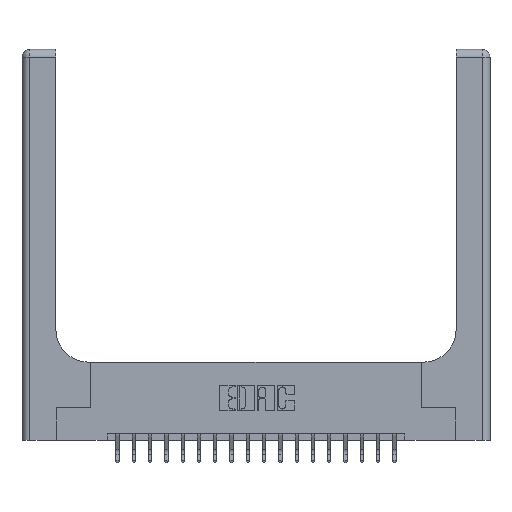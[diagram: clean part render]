
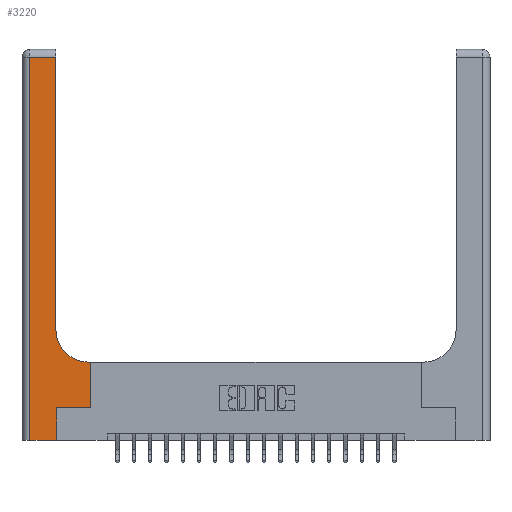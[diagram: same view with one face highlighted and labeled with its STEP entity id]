
A CAD part, top view. The second image highlights one B-rep face of the part: STEP entity #3220.
In plain terms, the highlighted planar face has unit normal (0, 0, 1).
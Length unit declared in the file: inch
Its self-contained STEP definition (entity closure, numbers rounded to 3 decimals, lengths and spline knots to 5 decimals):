
#283 = VERTEX_POINT ( 'NONE', #16008 ) ;
#293 = CARTESIAN_POINT ( 'NONE',  ( 0.51, 0.6, 0.37 ) ) ;
#525 = DIRECTION ( 'NONE',  ( 1., 0., 0. ) ) ;
#760 = DIRECTION ( 'NONE',  ( -1., 0., 0. ) ) ;
#823 = VECTOR ( 'NONE', #4569, 39.37008 ) ;
#890 = EDGE_CURVE ( 'NONE', #11549, #8494, #15449, .T. ) ;
#1393 = EDGE_CURVE ( 'NONE', #13385, #9423, #1812, .T. ) ;
#1415 = DIRECTION ( 'NONE',  ( 1., 0., 0. ) ) ;
#1431 = CARTESIAN_POINT ( 'NONE',  ( 0., 2.94, 0.37 ) ) ;
#1812 = LINE ( 'NONE', #1431, #823 ) ;
#2253 = CIRCLE ( 'NONE', #16131, 0.25 ) ;
#2894 = DIRECTION ( 'NONE',  ( 0., 1., 0. ) ) ;
#3220 = ADVANCED_FACE ( 'NONE', ( #13397 ), #10741, .F. ) ;
#3382 = LINE ( 'NONE', #13489, #16966 ) ;
#3398 = EDGE_CURVE ( 'NONE', #19363, #19264, #2253, .T. ) ;
#3534 = CARTESIAN_POINT ( 'NONE',  ( 0.26, 2.94, 0.37 ) ) ;
#3695 = VECTOR ( 'NONE', #13557, 39.37008 ) ;
#4569 = DIRECTION ( 'NONE',  ( -1., 0., 0. ) ) ;
#5801 = CARTESIAN_POINT ( 'NONE',  ( 0., 3., 0.37 ) ) ;
#6006 = DIRECTION ( 'NONE',  ( 0., 0., -1. ) ) ;
#6201 = CARTESIAN_POINT ( 'NONE',  ( 0., 0., 0.37 ) ) ;
#6215 = DIRECTION ( 'NONE',  ( 1., 0., 0. ) ) ;
#6959 = EDGE_CURVE ( 'NONE', #8494, #16603, #14528, .T. ) ;
#7045 = ORIENTED_EDGE ( 'NONE', *, *, #890, .T. ) ;
#7109 = CARTESIAN_POINT ( 'NONE',  ( 0.06, 3., 0.37 ) ) ;
#7228 = VECTOR ( 'NONE', #17967, 39.37008 ) ;
#7435 = CARTESIAN_POINT ( 'NONE',  ( 0.528, 0.25, 0.37 ) ) ;
#7507 = VECTOR ( 'NONE', #10739, 39.37008 ) ;
#7674 = EDGE_CURVE ( 'NONE', #8928, #11549, #9984, .T. ) ;
#8494 = VERTEX_POINT ( 'NONE', #15177 ) ;
#8783 = VECTOR ( 'NONE', #1415, 39.37008 ) ;
#8928 = VERTEX_POINT ( 'NONE', #9923 ) ;
#9072 = ORIENTED_EDGE ( 'NONE', *, *, #3398, .T. ) ;
#9423 = VERTEX_POINT ( 'NONE', #20302 ) ;
#9435 = CARTESIAN_POINT ( 'NONE',  ( 0.26, 3., 0.37 ) ) ;
#9743 = EDGE_CURVE ( 'NONE', #9423, #283, #19953, .T. ) ;
#9748 = ORIENTED_EDGE ( 'NONE', *, *, #1393, .T. ) ;
#9895 = CARTESIAN_POINT ( 'NONE',  ( 0.265, 0., 0.37 ) ) ;
#9923 = CARTESIAN_POINT ( 'NONE',  ( 0.265, 0., 0.37 ) ) ;
#9984 = LINE ( 'NONE', #9895, #7228 ) ;
#10601 = DIRECTION ( 'NONE',  ( -1., 0., 0. ) ) ;
#10739 = DIRECTION ( 'NONE',  ( 0., 1., 0. ) ) ;
#10741 = PLANE ( 'NONE',  #14442 ) ;
#11025 = EDGE_CURVE ( 'NONE', #19264, #13385, #14865, .T. ) ;
#11232 = VECTOR ( 'NONE', #525, 39.37008 ) ;
#11294 = ORIENTED_EDGE ( 'NONE', *, *, #9743, .T. ) ;
#11509 = CARTESIAN_POINT ( 'NONE',  ( 0.265, 0.25, 0.37 ) ) ;
#11549 = VERTEX_POINT ( 'NONE', #18530 ) ;
#11647 = ORIENTED_EDGE ( 'NONE', *, *, #6959, .T. ) ;
#11654 = VECTOR ( 'NONE', #2894, 39.37008 ) ;
#11946 = ORIENTED_EDGE ( 'NONE', *, *, #11025, .T. ) ;
#13122 = ORIENTED_EDGE ( 'NONE', *, *, #7674, .T. ) ;
#13273 = EDGE_CURVE ( 'NONE', #283, #8928, #17973, .T. ) ;
#13385 = VERTEX_POINT ( 'NONE', #3534 ) ;
#13397 = FACE_OUTER_BOUND ( 'NONE', #18627, .T. ) ;
#13489 = CARTESIAN_POINT ( 'NONE',  ( 0.26, 0.6, 0.37 ) ) ;
#13557 = DIRECTION ( 'NONE',  ( 0., -1., 0. ) ) ;
#13669 = EDGE_CURVE ( 'NONE', #16603, #19363, #3382, .T. ) ;
#14156 = DIRECTION ( 'NONE',  ( 0., 0., -1. ) ) ;
#14442 = AXIS2_PLACEMENT_3D ( 'NONE', #5801, #6006, #10601 ) ;
#14528 = LINE ( 'NONE', #7435, #7507 ) ;
#14865 = LINE ( 'NONE', #9435, #11654 ) ;
#15177 = CARTESIAN_POINT ( 'NONE',  ( 0.528, 0.25, 0.37 ) ) ;
#15449 = LINE ( 'NONE', #11509, #11232 ) ;
#15782 = ORIENTED_EDGE ( 'NONE', *, *, #13669, .T. ) ;
#16008 = CARTESIAN_POINT ( 'NONE',  ( 0.06, 0., 0.37 ) ) ;
#16131 = AXIS2_PLACEMENT_3D ( 'NONE', #20328, #14156, #6215 ) ;
#16603 = VERTEX_POINT ( 'NONE', #17823 ) ;
#16966 = VECTOR ( 'NONE', #760, 39.37008 ) ;
#17288 = CARTESIAN_POINT ( 'NONE',  ( 0.26, 0.85, 0.37 ) ) ;
#17823 = CARTESIAN_POINT ( 'NONE',  ( 0.528, 0.6, 0.37 ) ) ;
#17967 = DIRECTION ( 'NONE',  ( 0., 1., 0. ) ) ;
#17973 = LINE ( 'NONE', #6201, #8783 ) ;
#18530 = CARTESIAN_POINT ( 'NONE',  ( 0.265, 0.25, 0.37 ) ) ;
#18627 = EDGE_LOOP ( 'NONE', ( #11946, #9748, #11294, #20071, #13122, #7045, #11647, #15782, #9072 ) ) ;
#19264 = VERTEX_POINT ( 'NONE', #17288 ) ;
#19363 = VERTEX_POINT ( 'NONE', #293 ) ;
#19953 = LINE ( 'NONE', #7109, #3695 ) ;
#20071 = ORIENTED_EDGE ( 'NONE', *, *, #13273, .T. ) ;
#20302 = CARTESIAN_POINT ( 'NONE',  ( 0.06, 2.94, 0.37 ) ) ;
#20328 = CARTESIAN_POINT ( 'NONE',  ( 0.51, 0.85, 0.37 ) ) ;
